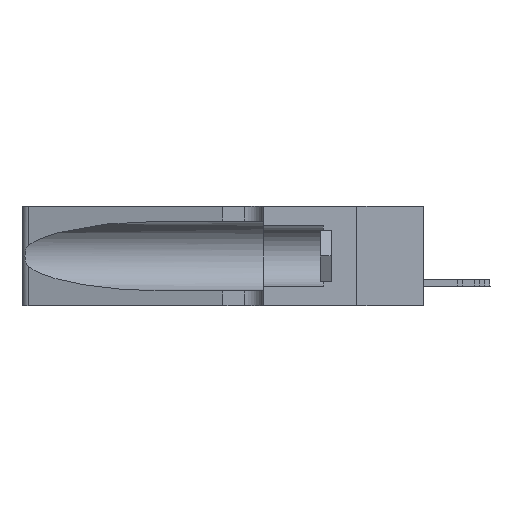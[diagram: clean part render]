
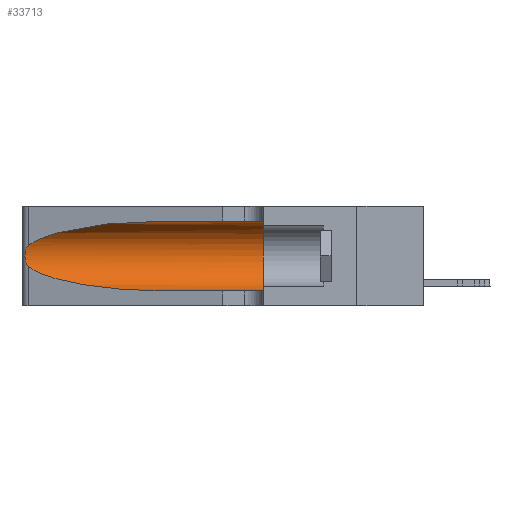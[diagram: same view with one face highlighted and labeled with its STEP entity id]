
A CAD part, left-side view. The second image highlights one B-rep face of the part: STEP entity #33713.
In plain terms, the highlighted cylindrical face has radius 3.308 mm (diameter 6.617 mm), a partial arc.
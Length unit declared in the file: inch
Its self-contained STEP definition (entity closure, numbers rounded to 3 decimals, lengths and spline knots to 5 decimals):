
#1112 = CARTESIAN_POINT ( 'NONE',  ( 0.25555, 1.22994, 0.2215 ) ) ;
#1252 = DIRECTION ( 'NONE',  ( 0., -1., 0. ) ) ;
#1265 = CARTESIAN_POINT ( 'NONE',  ( 0.25787, 1.23484, 0.2124 ) ) ;
#1279 = CARTESIAN_POINT ( 'NONE',  ( 0.26017, 1.23833, 0.17102 ) ) ;
#1402 = CARTESIAN_POINT ( 'NONE',  ( 0.1305, 1.61858, 0.31525 ) ) ;
#1500 = CARTESIAN_POINT ( 'NONE',  ( 0.2373, 1.15595, 0.08982 ) ) ;
#2580 = EDGE_LOOP ( 'NONE', ( #28725, #25407, #37020, #14255, #6087, #13304 ) ) ;
#2652 = DIRECTION ( 'NONE',  ( 0., 0., -1. ) ) ;
#2835 = CARTESIAN_POINT ( 'NONE',  ( 0.2373, 1.15595, 0.28018 ) ) ;
#3054 = CARTESIAN_POINT ( 'NONE',  ( 0.25639, 1.23186, 0.15144 ) ) ;
#3798 = EDGE_CURVE ( 'NONE', #6212, #41570, #27188, .T. ) ;
#4988 = CARTESIAN_POINT ( 'NONE',  ( 0.25487, 1.22718, 0.14631 ) ) ;
#5404 = CYLINDRICAL_SURFACE ( 'NONE', #26858, 0.13025 ) ;
#5471 = CARTESIAN_POINT ( 'NONE',  ( 0.25639, 1.23184, 0.21858 ) ) ;
#6087 = ORIENTED_EDGE ( 'NONE', *, *, #26851, .F. ) ;
#6212 = VERTEX_POINT ( 'NONE', #6794 ) ;
#6794 = CARTESIAN_POINT ( 'NONE',  ( 0.25487, 1.22718, 0.14631 ) ) ;
#8043 = FACE_OUTER_BOUND ( 'NONE', #2580, .T. ) ;
#8411 = CARTESIAN_POINT ( 'NONE',  ( 0.26075, 1.23896, 0.178 ) ) ;
#8454 = CARTESIAN_POINT ( 'NONE',  ( 0.25487, 1.22718, 0.22369 ) ) ;
#8642 = CARTESIAN_POINT ( 'NONE',  ( 0.1305, 0.35, 0.31525 ) ) ;
#10352 = CARTESIAN_POINT ( 'NONE',  ( 0.25487, 1.22718, 0.22369 ) ) ;
#10635 = DIRECTION ( 'NONE',  ( 0., 1., 0. ) ) ;
#10656 = B_SPLINE_CURVE_WITH_KNOTS ( 'NONE', 3,
 ( #40918, #1112, #5471, #1265, #21995, #28233, #11484, #8411, #1279, #47277, #10765, #3054, #38988, #35483 ),
 .UNSPECIFIED., .F., .F.,
 ( 4, 2, 2, 2, 2, 2, 4 ),
 ( 0., 0.00027, 0.00053, 0.00107, 0.0016, 0.00187, 0.00214 ),
 .UNSPECIFIED. ) ;
#10765 = CARTESIAN_POINT ( 'NONE',  ( 0.25789, 1.23486, 0.15765 ) ) ;
#11484 = CARTESIAN_POINT ( 'NONE',  ( 0.26075, 1.23896, 0.19203 ) ) ;
#13049 = CARTESIAN_POINT ( 'NONE',  ( 0.18966, 0.96281, 0.05475 ) ) ;
#13304 = ORIENTED_EDGE ( 'NONE', *, *, #22572, .F. ) ;
#14097 = EDGE_CURVE ( 'NONE', #41740, #20607, #46502, .T. ) ;
#14209 = LINE ( 'NONE', #1402, #47737 ) ;
#14255 = ORIENTED_EDGE ( 'NONE', *, *, #49714, .T. ) ;
#17524 = DIRECTION ( 'NONE',  ( 0., -1., 0. ) ) ;
#18624 = CARTESIAN_POINT ( 'NONE',  ( 0.1305, 0.35, 0.05475 ) ) ;
#18638 = VECTOR ( 'NONE', #27154, 39.37008 ) ;
#20253 = EDGE_CURVE ( 'NONE', #20607, #6212, #10656, .T. ) ;
#20607 = VERTEX_POINT ( 'NONE', #8454 ) ;
#21995 = CARTESIAN_POINT ( 'NONE',  ( 0.25854, 1.2359, 0.20912 ) ) ;
#22572 = EDGE_CURVE ( 'NONE', #41740, #46892, #14209, .T. ) ;
#25407 = ORIENTED_EDGE ( 'NONE', *, *, #20253, .T. ) ;
#26596 = CARTESIAN_POINT ( 'NONE',  ( 0.18966, 0.96281, 0.31525 ) ) ;
#26851 = EDGE_CURVE ( 'NONE', #46892, #30885, #49657, .T. ) ;
#26858 = AXIS2_PLACEMENT_3D ( 'NONE', #40871, #1252, #2652 ) ;
#27154 = DIRECTION ( 'NONE',  ( 0., -1., 0. ) ) ;
#27188 =( BOUNDED_CURVE ( )  B_SPLINE_CURVE ( 3, ( #4988, #1500, #13049, #33333 ),
 .UNSPECIFIED., .F., .F. ) 
 B_SPLINE_CURVE_WITH_KNOTS ( ( 4, 4 ),
 ( 3.44316, 4.71239 ),
 .UNSPECIFIED. ) 
 CURVE ( )  GEOMETRIC_REPRESENTATION_ITEM ( )  RATIONAL_B_SPLINE_CURVE ( ( 1., 0.87, 0.87, 1. ) ) 
 REPRESENTATION_ITEM ( '' )  );
#28233 = CARTESIAN_POINT ( 'NONE',  ( 0.26018, 1.23835, 0.19895 ) ) ;
#28725 = ORIENTED_EDGE ( 'NONE', *, *, #14097, .T. ) ;
#30515 = DIRECTION ( 'NONE',  ( 0., 0., 1. ) ) ;
#30885 = VERTEX_POINT ( 'NONE', #18624 ) ;
#33333 = CARTESIAN_POINT ( 'NONE',  ( 0.1305, 0.72297, 0.05475 ) ) ;
#33713 = ADVANCED_FACE ( 'NONE', ( #8043 ), #5404, .F. ) ;
#34519 = CARTESIAN_POINT ( 'NONE',  ( 0.1305, 0.72297, 0.31525 ) ) ;
#35483 = CARTESIAN_POINT ( 'NONE',  ( 0.25487, 1.22718, 0.14631 ) ) ;
#37020 = ORIENTED_EDGE ( 'NONE', *, *, #3798, .T. ) ;
#38576 = CARTESIAN_POINT ( 'NONE',  ( 0.1305, 0.72297, 0.31525 ) ) ;
#38988 = CARTESIAN_POINT ( 'NONE',  ( 0.25555, 1.22993, 0.14849 ) ) ;
#40711 = LINE ( 'NONE', #47576, #18638 ) ;
#40871 = CARTESIAN_POINT ( 'NONE',  ( 0.1305, 1.61858, 0.185 ) ) ;
#40918 = CARTESIAN_POINT ( 'NONE',  ( 0.25487, 1.22718, 0.22369 ) ) ;
#41570 = VERTEX_POINT ( 'NONE', #49001 ) ;
#41740 = VERTEX_POINT ( 'NONE', #38576 ) ;
#42495 = CARTESIAN_POINT ( 'NONE',  ( 0.1305, 0.35, 0.185 ) ) ;
#46139 = AXIS2_PLACEMENT_3D ( 'NONE', #42495, #10635, #30515 ) ;
#46502 =( BOUNDED_CURVE ( )  B_SPLINE_CURVE ( 3, ( #34519, #26596, #2835, #10352 ),
 .UNSPECIFIED., .F., .T. ) 
 B_SPLINE_CURVE_WITH_KNOTS ( ( 4, 4 ),
 ( 1.5708, 2.84003 ),
 .UNSPECIFIED. ) 
 CURVE ( )  GEOMETRIC_REPRESENTATION_ITEM ( )  RATIONAL_B_SPLINE_CURVE ( ( 1., 0.87, 0.87, 1. ) ) 
 REPRESENTATION_ITEM ( '' )  );
#46892 = VERTEX_POINT ( 'NONE', #8642 ) ;
#47277 = CARTESIAN_POINT ( 'NONE',  ( 0.25856, 1.23593, 0.16098 ) ) ;
#47576 = CARTESIAN_POINT ( 'NONE',  ( 0.1305, 1.61858, 0.05475 ) ) ;
#47737 = VECTOR ( 'NONE', #17524, 39.37008 ) ;
#49001 = CARTESIAN_POINT ( 'NONE',  ( 0.1305, 0.72297, 0.05475 ) ) ;
#49657 = CIRCLE ( 'NONE', #46139, 0.13025 ) ;
#49714 = EDGE_CURVE ( 'NONE', #41570, #30885, #40711, .T. ) ;
